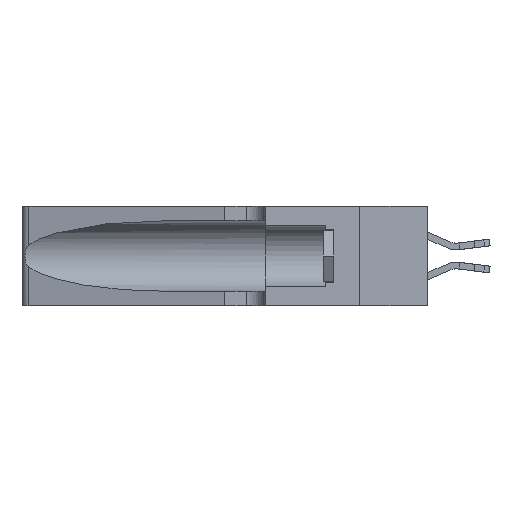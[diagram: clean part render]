
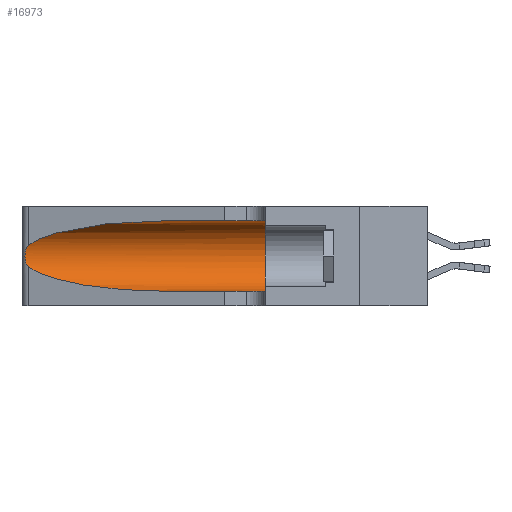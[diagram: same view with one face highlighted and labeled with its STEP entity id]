
A CAD part, left-side view. The second image highlights one B-rep face of the part: STEP entity #16973.
In plain terms, the highlighted cylindrical face has radius 3.308 mm (diameter 6.617 mm), a partial arc.
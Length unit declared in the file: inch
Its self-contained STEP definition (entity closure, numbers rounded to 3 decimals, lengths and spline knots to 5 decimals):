
#68 = EDGE_LOOP ( 'NONE', ( #29563, #30459, #17129, #32239, #12169, #34879 ) ) ;
#264 = CARTESIAN_POINT ( 'NONE',  ( 0.1305, 0.35, 0.05475 ) ) ;
#377 = CARTESIAN_POINT ( 'NONE',  ( 0.1305, 0.35, 0.185 ) ) ;
#954 = CARTESIAN_POINT ( 'NONE',  ( 0.1305, 1.61858, 0.31525 ) ) ;
#1675 = DIRECTION ( 'NONE',  ( 0., -1., 0. ) ) ;
#2030 = CARTESIAN_POINT ( 'NONE',  ( 0.25487, 1.22718, 0.14631 ) ) ;
#2238 = EDGE_CURVE ( 'NONE', #10264, #5534, #12583, .T. ) ;
#2513 = EDGE_CURVE ( 'NONE', #5398, #24858, #17471, .T. ) ;
#3446 = DIRECTION ( 'NONE',  ( 0., 0., 1. ) ) ;
#4383 = CARTESIAN_POINT ( 'NONE',  ( 0.1305, 0.72297, 0.05475 ) ) ;
#4910 = CARTESIAN_POINT ( 'NONE',  ( 0.25487, 1.22718, 0.22369 ) ) ;
#5398 = VERTEX_POINT ( 'NONE', #23755 ) ;
#5534 = VERTEX_POINT ( 'NONE', #24471 ) ;
#5898 = CARTESIAN_POINT ( 'NONE',  ( 0.1305, 0.72297, 0.05475 ) ) ;
#5907 = CARTESIAN_POINT ( 'NONE',  ( 0.1305, 1.61858, 0.185 ) ) ;
#6927 =( BOUNDED_CURVE ( )  B_SPLINE_CURVE ( 3, ( #18254, #9533, #15493, #35340 ),
 .UNSPECIFIED., .F., .F. ) 
 B_SPLINE_CURVE_WITH_KNOTS ( ( 4, 4 ),
 ( 1.5708, 2.84003 ),
 .UNSPECIFIED. ) 
 CURVE ( )  GEOMETRIC_REPRESENTATION_ITEM ( )  RATIONAL_B_SPLINE_CURVE ( ( 1., 0.87, 0.87, 1. ) ) 
 REPRESENTATION_ITEM ( '' )  );
#7919 = CARTESIAN_POINT ( 'NONE',  ( 0.25854, 1.2359, 0.20912 ) ) ;
#8354 = VECTOR ( 'NONE', #9891, 39.37008 ) ;
#9276 = LINE ( 'NONE', #954, #8354 ) ;
#9533 = CARTESIAN_POINT ( 'NONE',  ( 0.18966, 0.96281, 0.31525 ) ) ;
#9891 = DIRECTION ( 'NONE',  ( 0., -1., 0. ) ) ;
#10264 = VERTEX_POINT ( 'NONE', #34166 ) ;
#10912 = CARTESIAN_POINT ( 'NONE',  ( 0.26075, 1.23896, 0.19203 ) ) ;
#10965 =( BOUNDED_CURVE ( )  B_SPLINE_CURVE ( 3, ( #17536, #11738, #23254, #5898 ),
 .UNSPECIFIED., .F., .F. ) 
 B_SPLINE_CURVE_WITH_KNOTS ( ( 4, 4 ),
 ( 3.44316, 4.71239 ),
 .UNSPECIFIED. ) 
 CURVE ( )  GEOMETRIC_REPRESENTATION_ITEM ( )  RATIONAL_B_SPLINE_CURVE ( ( 1., 0.87, 0.87, 1. ) ) 
 REPRESENTATION_ITEM ( '' )  );
#11738 = CARTESIAN_POINT ( 'NONE',  ( 0.2373, 1.15595, 0.08982 ) ) ;
#12169 = ORIENTED_EDGE ( 'NONE', *, *, #2513, .F. ) ;
#12583 = B_SPLINE_CURVE_WITH_KNOTS ( 'NONE', 3,
 ( #4910, #22325, #19471, #25148, #7919, #27999, #10912, #30880, #13798, #33710, #16704, #36524, #19593, #2030 ),
 .UNSPECIFIED., .F., .F.,
 ( 4, 2, 2, 2, 2, 2, 4 ),
 ( 0., 0.00027, 0.00053, 0.00107, 0.0016, 0.00187, 0.00214 ),
 .UNSPECIFIED. ) ;
#12696 = EDGE_CURVE ( 'NONE', #13619, #24858, #36120, .T. ) ;
#13170 = CYLINDRICAL_SURFACE ( 'NONE', #16782, 0.13025 ) ;
#13523 = EDGE_CURVE ( 'NONE', #31707, #5398, #9276, .T. ) ;
#13619 = VERTEX_POINT ( 'NONE', #4383 ) ;
#13798 = CARTESIAN_POINT ( 'NONE',  ( 0.26017, 1.23833, 0.17102 ) ) ;
#15493 = CARTESIAN_POINT ( 'NONE',  ( 0.2373, 1.15595, 0.28018 ) ) ;
#16704 = CARTESIAN_POINT ( 'NONE',  ( 0.25789, 1.23486, 0.15765 ) ) ;
#16782 = AXIS2_PLACEMENT_3D ( 'NONE', #5907, #26095, #23267 ) ;
#16973 = ADVANCED_FACE ( 'NONE', ( #35841 ), #13170, .F. ) ;
#17129 = ORIENTED_EDGE ( 'NONE', *, *, #31271, .T. ) ;
#17471 = CIRCLE ( 'NONE', #27099, 0.13025 ) ;
#17536 = CARTESIAN_POINT ( 'NONE',  ( 0.25487, 1.22718, 0.14631 ) ) ;
#18254 = CARTESIAN_POINT ( 'NONE',  ( 0.1305, 0.72297, 0.31525 ) ) ;
#19471 = CARTESIAN_POINT ( 'NONE',  ( 0.25639, 1.23184, 0.21858 ) ) ;
#19593 = CARTESIAN_POINT ( 'NONE',  ( 0.25555, 1.22993, 0.14849 ) ) ;
#20924 = DIRECTION ( 'NONE',  ( 0., 1., 0. ) ) ;
#22325 = CARTESIAN_POINT ( 'NONE',  ( 0.25555, 1.22994, 0.2215 ) ) ;
#23254 = CARTESIAN_POINT ( 'NONE',  ( 0.18966, 0.96281, 0.05475 ) ) ;
#23267 = DIRECTION ( 'NONE',  ( 0., 0., -1. ) ) ;
#23755 = CARTESIAN_POINT ( 'NONE',  ( 0.1305, 0.35, 0.31525 ) ) ;
#24306 = EDGE_CURVE ( 'NONE', #31707, #10264, #6927, .T. ) ;
#24471 = CARTESIAN_POINT ( 'NONE',  ( 0.25487, 1.22718, 0.14631 ) ) ;
#24792 = CARTESIAN_POINT ( 'NONE',  ( 0.1305, 0.72297, 0.31525 ) ) ;
#24858 = VERTEX_POINT ( 'NONE', #264 ) ;
#25148 = CARTESIAN_POINT ( 'NONE',  ( 0.25787, 1.23484, 0.2124 ) ) ;
#26095 = DIRECTION ( 'NONE',  ( 0., -1., 0. ) ) ;
#27099 = AXIS2_PLACEMENT_3D ( 'NONE', #377, #20924, #3446 ) ;
#27666 = CARTESIAN_POINT ( 'NONE',  ( 0.1305, 1.61858, 0.05475 ) ) ;
#27999 = CARTESIAN_POINT ( 'NONE',  ( 0.26018, 1.23835, 0.19895 ) ) ;
#29563 = ORIENTED_EDGE ( 'NONE', *, *, #24306, .T. ) ;
#30459 = ORIENTED_EDGE ( 'NONE', *, *, #2238, .T. ) ;
#30880 = CARTESIAN_POINT ( 'NONE',  ( 0.26075, 1.23896, 0.178 ) ) ;
#31271 = EDGE_CURVE ( 'NONE', #5534, #13619, #10965, .T. ) ;
#31707 = VERTEX_POINT ( 'NONE', #24792 ) ;
#32239 = ORIENTED_EDGE ( 'NONE', *, *, #12696, .T. ) ;
#33710 = CARTESIAN_POINT ( 'NONE',  ( 0.25856, 1.23593, 0.16098 ) ) ;
#34166 = CARTESIAN_POINT ( 'NONE',  ( 0.25487, 1.22718, 0.22369 ) ) ;
#34879 = ORIENTED_EDGE ( 'NONE', *, *, #13523, .F. ) ;
#35250 = VECTOR ( 'NONE', #1675, 39.37008 ) ;
#35340 = CARTESIAN_POINT ( 'NONE',  ( 0.25487, 1.22718, 0.22369 ) ) ;
#35841 = FACE_OUTER_BOUND ( 'NONE', #68, .T. ) ;
#36120 = LINE ( 'NONE', #27666, #35250 ) ;
#36524 = CARTESIAN_POINT ( 'NONE',  ( 0.25639, 1.23186, 0.15144 ) ) ;
